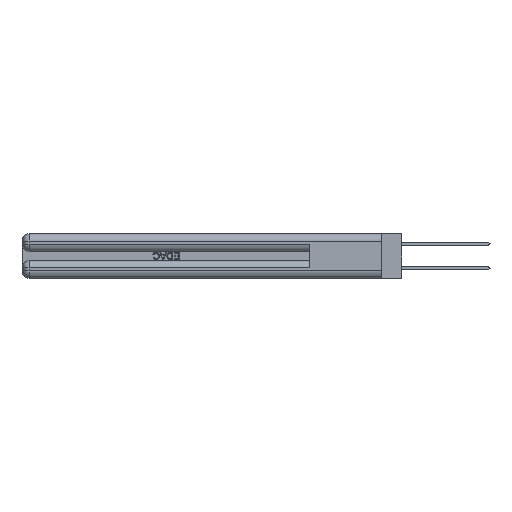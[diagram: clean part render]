
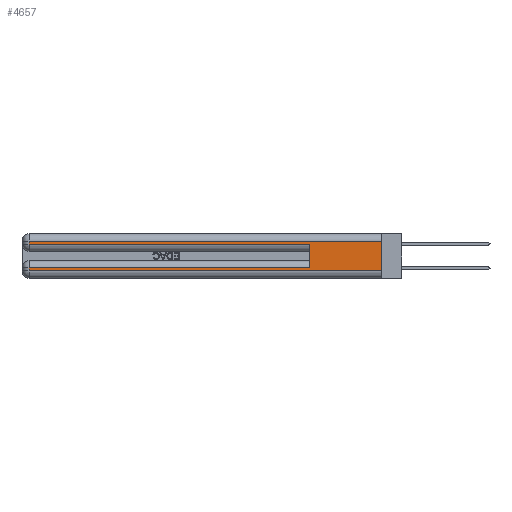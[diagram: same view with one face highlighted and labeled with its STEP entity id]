
A CAD part, left-side view. The second image highlights one B-rep face of the part: STEP entity #4657.
In plain terms, the highlighted planar face has unit normal (-1, 0, 0).
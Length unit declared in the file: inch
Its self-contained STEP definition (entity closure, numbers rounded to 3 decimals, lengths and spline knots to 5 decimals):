
#46 = DIRECTION ( 'NONE',  ( 1., 0., 0. ) ) ;
#172 = DIRECTION ( 'NONE',  ( 0., -1., 0. ) ) ;
#360 = CARTESIAN_POINT ( 'NONE',  ( 0., 2.94, 0.31 ) ) ;
#465 = VECTOR ( 'NONE', #23681, 39.37008 ) ;
#1172 = LINE ( 'NONE', #4569, #34640 ) ;
#1303 = EDGE_CURVE ( 'NONE', #21933, #36039, #24908, .T. ) ;
#1480 = CARTESIAN_POINT ( 'NONE',  ( 0., 2.94, 0.085 ) ) ;
#2153 = VERTEX_POINT ( 'NONE', #19753 ) ;
#3230 = CARTESIAN_POINT ( 'NONE',  ( 0., 2.94, 0.37 ) ) ;
#4434 = CARTESIAN_POINT ( 'NONE',  ( 0., 0., 0.37 ) ) ;
#4569 = CARTESIAN_POINT ( 'NONE',  ( 0., 0., 0.31 ) ) ;
#4657 = ADVANCED_FACE ( 'NONE', ( #14796 ), #12946, .F. ) ;
#4933 = CARTESIAN_POINT ( 'NONE',  ( 0., 2.94, 0.285 ) ) ;
#4943 = LINE ( 'NONE', #4434, #14566 ) ;
#5931 = LINE ( 'NONE', #11176, #37376 ) ;
#6357 = LINE ( 'NONE', #13071, #14960 ) ;
#7571 = CARTESIAN_POINT ( 'NONE',  ( 0., 0., 0.085 ) ) ;
#7924 = VERTEX_POINT ( 'NONE', #360 ) ;
#8290 = VERTEX_POINT ( 'NONE', #38352 ) ;
#8926 = LINE ( 'NONE', #3230, #34795 ) ;
#9673 = CARTESIAN_POINT ( 'NONE',  ( 0., 0., 0.37 ) ) ;
#10982 = VERTEX_POINT ( 'NONE', #1480 ) ;
#11176 = CARTESIAN_POINT ( 'NONE',  ( 0., 2.94, 0.37 ) ) ;
#12045 = VERTEX_POINT ( 'NONE', #4933 ) ;
#12210 = ORIENTED_EDGE ( 'NONE', *, *, #1303, .F. ) ;
#12946 = PLANE ( 'NONE',  #33942 ) ;
#13071 = CARTESIAN_POINT ( 'NONE',  ( 0., 0., 0.06 ) ) ;
#14453 = DIRECTION ( 'NONE',  ( 0., 0., -1. ) ) ;
#14566 = VECTOR ( 'NONE', #23803, 39.37008 ) ;
#14796 = FACE_OUTER_BOUND ( 'NONE', #37402, .T. ) ;
#14802 = CARTESIAN_POINT ( 'NONE',  ( 0., 0.6, 0.285 ) ) ;
#14960 = VECTOR ( 'NONE', #172, 39.37008 ) ;
#18698 = CARTESIAN_POINT ( 'NONE',  ( 0., 2.94, 0.06 ) ) ;
#19753 = CARTESIAN_POINT ( 'NONE',  ( 0., 0., 0.31 ) ) ;
#20966 = EDGE_CURVE ( 'NONE', #2153, #7924, #1172, .T. ) ;
#21217 = VERTEX_POINT ( 'NONE', #18698 ) ;
#21533 = ORIENTED_EDGE ( 'NONE', *, *, #32578, .F. ) ;
#21933 = VERTEX_POINT ( 'NONE', #41658 ) ;
#22441 = ORIENTED_EDGE ( 'NONE', *, *, #20966, .T. ) ;
#22683 = DIRECTION ( 'NONE',  ( 0., 0., -1. ) ) ;
#23029 = EDGE_CURVE ( 'NONE', #21933, #10982, #34980, .T. ) ;
#23477 = EDGE_CURVE ( 'NONE', #21217, #8290, #6357, .T. ) ;
#23681 = DIRECTION ( 'NONE',  ( 0., 1., 0. ) ) ;
#23803 = DIRECTION ( 'NONE',  ( 0., 0., -1. ) ) ;
#23861 = CARTESIAN_POINT ( 'NONE',  ( 0., 0.6, 0.145 ) ) ;
#24908 = LINE ( 'NONE', #23861, #41205 ) ;
#25807 = DIRECTION ( 'NONE',  ( 0., -1., 0. ) ) ;
#25885 = DIRECTION ( 'NONE',  ( 0., 0., -1. ) ) ;
#26575 = ORIENTED_EDGE ( 'NONE', *, *, #26804, .T. ) ;
#26804 = EDGE_CURVE ( 'NONE', #12045, #36039, #38562, .T. ) ;
#29415 = EDGE_CURVE ( 'NONE', #10982, #21217, #5931, .T. ) ;
#29738 = EDGE_CURVE ( 'NONE', #7924, #12045, #8926, .T. ) ;
#29875 = VECTOR ( 'NONE', #25807, 39.37008 ) ;
#30929 = ORIENTED_EDGE ( 'NONE', *, *, #29415, .T. ) ;
#32578 = EDGE_CURVE ( 'NONE', #2153, #8290, #4943, .T. ) ;
#33942 = AXIS2_PLACEMENT_3D ( 'NONE', #9673, #46, #22683 ) ;
#34640 = VECTOR ( 'NONE', #40316, 39.37008 ) ;
#34795 = VECTOR ( 'NONE', #25885, 39.37008 ) ;
#34903 = ORIENTED_EDGE ( 'NONE', *, *, #23477, .T. ) ;
#34980 = LINE ( 'NONE', #7571, #465 ) ;
#36003 = ORIENTED_EDGE ( 'NONE', *, *, #23029, .T. ) ;
#36039 = VERTEX_POINT ( 'NONE', #14802 ) ;
#36955 = DIRECTION ( 'NONE',  ( 0., 0., 1. ) ) ;
#37376 = VECTOR ( 'NONE', #14453, 39.37008 ) ;
#37402 = EDGE_LOOP ( 'NONE', ( #21533, #22441, #40616, #26575, #12210, #36003, #30929, #34903 ) ) ;
#38352 = CARTESIAN_POINT ( 'NONE',  ( 0., 0., 0.06 ) ) ;
#38562 = LINE ( 'NONE', #38771, #29875 ) ;
#38771 = CARTESIAN_POINT ( 'NONE',  ( 0., 0., 0.285 ) ) ;
#40316 = DIRECTION ( 'NONE',  ( 0., 1., 0. ) ) ;
#40616 = ORIENTED_EDGE ( 'NONE', *, *, #29738, .T. ) ;
#41205 = VECTOR ( 'NONE', #36955, 39.37008 ) ;
#41658 = CARTESIAN_POINT ( 'NONE',  ( 0., 0.6, 0.085 ) ) ;
